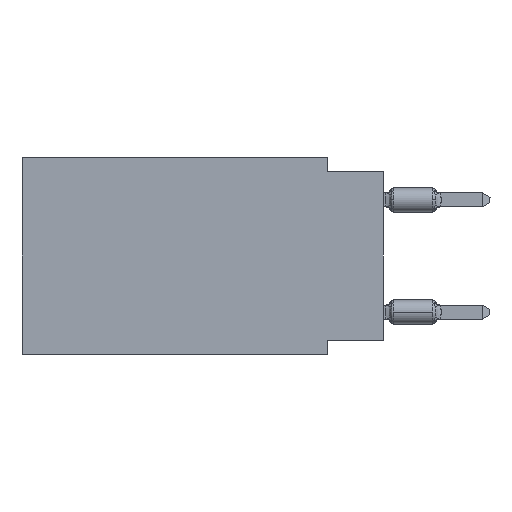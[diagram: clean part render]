
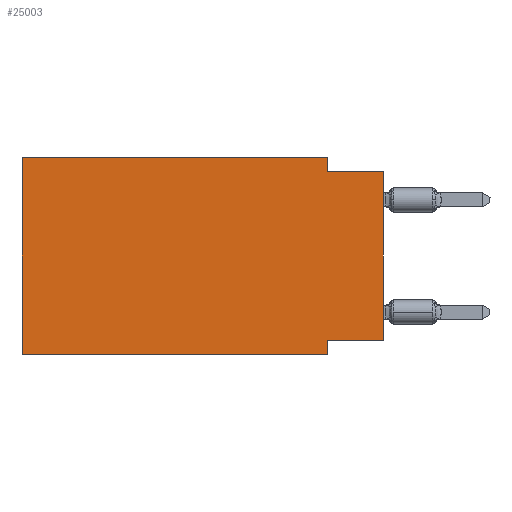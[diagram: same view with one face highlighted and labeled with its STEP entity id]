
A CAD part, left-side view. The second image highlights one B-rep face of the part: STEP entity #25003.
In plain terms, the highlighted planar face has unit normal (-1, 0, 0).
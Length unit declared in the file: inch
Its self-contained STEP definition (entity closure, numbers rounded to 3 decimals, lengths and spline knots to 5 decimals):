
#444 = ORIENTED_EDGE ( 'NONE', *, *, #64696, .F. ) ;
#551 = LINE ( 'NONE', #21328, #1518 ) ;
#741 = CARTESIAN_POINT ( 'NONE',  ( 0., 0.645, 0. ) ) ;
#1518 = VECTOR ( 'NONE', #42098, 39.37008 ) ;
#2371 = ORIENTED_EDGE ( 'NONE', *, *, #37936, .T. ) ;
#2603 = EDGE_CURVE ( 'NONE', #9441, #37464, #52927, .T. ) ;
#3556 = CARTESIAN_POINT ( 'NONE',  ( 0., 0., -0.025 ) ) ;
#4862 = DIRECTION ( 'NONE',  ( 0., 0., -1. ) ) ;
#5834 = LINE ( 'NONE', #741, #36054 ) ;
#6210 = VERTEX_POINT ( 'NONE', #25423 ) ;
#6483 = FACE_OUTER_BOUND ( 'NONE', #27302, .T. ) ;
#8484 = DIRECTION ( 'NONE',  ( 0., 0., 1. ) ) ;
#8625 = LINE ( 'NONE', #18156, #59385 ) ;
#9027 = DIRECTION ( 'NONE',  ( 0., -1., 0. ) ) ;
#9147 = CARTESIAN_POINT ( 'NONE',  ( 0., 0.1, -0.025 ) ) ;
#9367 = LINE ( 'NONE', #3556, #36506 ) ;
#9441 = VERTEX_POINT ( 'NONE', #24440 ) ;
#9994 = LINE ( 'NONE', #30731, #37786 ) ;
#12358 = DIRECTION ( 'NONE',  ( 0., -1., 0. ) ) ;
#14740 = EDGE_CURVE ( 'NONE', #63512, #6210, #8625, .T. ) ;
#15233 = VECTOR ( 'NONE', #52269, 39.37008 ) ;
#15300 = CARTESIAN_POINT ( 'NONE',  ( 0., 0., -0.025 ) ) ;
#16416 = DIRECTION ( 'NONE',  ( 0., -1., 0. ) ) ;
#16807 = EDGE_CURVE ( 'NONE', #35887, #25252, #9367, .T. ) ;
#17049 = DIRECTION ( 'NONE',  ( 1., 0., 0. ) ) ;
#17798 = AXIS2_PLACEMENT_3D ( 'NONE', #42566, #17049, #37122 ) ;
#18156 = CARTESIAN_POINT ( 'NONE',  ( 0., 0.645, -0.35 ) ) ;
#19279 = ORIENTED_EDGE ( 'NONE', *, *, #2603, .F. ) ;
#21328 = CARTESIAN_POINT ( 'NONE',  ( 0., 0.1, -0.35 ) ) ;
#21627 = VERTEX_POINT ( 'NONE', #41822 ) ;
#23287 = CARTESIAN_POINT ( 'NONE',  ( 0., 0.1, 0. ) ) ;
#24440 = CARTESIAN_POINT ( 'NONE',  ( 0., 0., -0.325 ) ) ;
#25003 = ADVANCED_FACE ( 'NONE', ( #6483 ), #53472, .F. ) ;
#25252 = VERTEX_POINT ( 'NONE', #15300 ) ;
#25423 = CARTESIAN_POINT ( 'NONE',  ( 0., 0.1, -0.35 ) ) ;
#27302 = EDGE_LOOP ( 'NONE', ( #2371, #36614, #49413, #444, #40631, #62950, #48847, #19279 ) ) ;
#27366 = CARTESIAN_POINT ( 'NONE',  ( 0., 0., -0.325 ) ) ;
#30731 = CARTESIAN_POINT ( 'NONE',  ( 0., 0.1, 0. ) ) ;
#32671 = EDGE_CURVE ( 'NONE', #63512, #21627, #50356, .T. ) ;
#33338 = VERTEX_POINT ( 'NONE', #23287 ) ;
#33691 = EDGE_CURVE ( 'NONE', #33338, #35887, #9994, .T. ) ;
#33709 = VECTOR ( 'NONE', #53203, 39.37008 ) ;
#35887 = VERTEX_POINT ( 'NONE', #9147 ) ;
#36054 = VECTOR ( 'NONE', #16416, 39.37008 ) ;
#36506 = VECTOR ( 'NONE', #9027, 39.37008 ) ;
#36560 = VECTOR ( 'NONE', #8484, 39.37008 ) ;
#36614 = ORIENTED_EDGE ( 'NONE', *, *, #16807, .F. ) ;
#37122 = DIRECTION ( 'NONE',  ( 0., 0., -1. ) ) ;
#37464 = VERTEX_POINT ( 'NONE', #61858 ) ;
#37786 = VECTOR ( 'NONE', #4862, 39.37008 ) ;
#37936 = EDGE_CURVE ( 'NONE', #9441, #25252, #48750, .T. ) ;
#38394 = CARTESIAN_POINT ( 'NONE',  ( 0., 0.645, -0.35 ) ) ;
#40631 = ORIENTED_EDGE ( 'NONE', *, *, #32671, .F. ) ;
#41822 = CARTESIAN_POINT ( 'NONE',  ( 0., 0.645, 0. ) ) ;
#42098 = DIRECTION ( 'NONE',  ( 0., 0., -1. ) ) ;
#42566 = CARTESIAN_POINT ( 'NONE',  ( 0., 0.645, 0. ) ) ;
#43974 = CARTESIAN_POINT ( 'NONE',  ( 0., 0., 0. ) ) ;
#44390 = EDGE_CURVE ( 'NONE', #37464, #6210, #551, .T. ) ;
#46234 = CARTESIAN_POINT ( 'NONE',  ( 0., 0.645, 0. ) ) ;
#48750 = LINE ( 'NONE', #43974, #33709 ) ;
#48847 = ORIENTED_EDGE ( 'NONE', *, *, #44390, .F. ) ;
#49413 = ORIENTED_EDGE ( 'NONE', *, *, #33691, .F. ) ;
#50356 = LINE ( 'NONE', #46234, #36560 ) ;
#52269 = DIRECTION ( 'NONE',  ( 0., 1., 0. ) ) ;
#52927 = LINE ( 'NONE', #27366, #15233 ) ;
#53203 = DIRECTION ( 'NONE',  ( 0., 0., 1. ) ) ;
#53472 = PLANE ( 'NONE',  #17798 ) ;
#59385 = VECTOR ( 'NONE', #12358, 39.37008 ) ;
#61858 = CARTESIAN_POINT ( 'NONE',  ( 0., 0.1, -0.325 ) ) ;
#62950 = ORIENTED_EDGE ( 'NONE', *, *, #14740, .T. ) ;
#63512 = VERTEX_POINT ( 'NONE', #38394 ) ;
#64696 = EDGE_CURVE ( 'NONE', #21627, #33338, #5834, .T. ) ;
